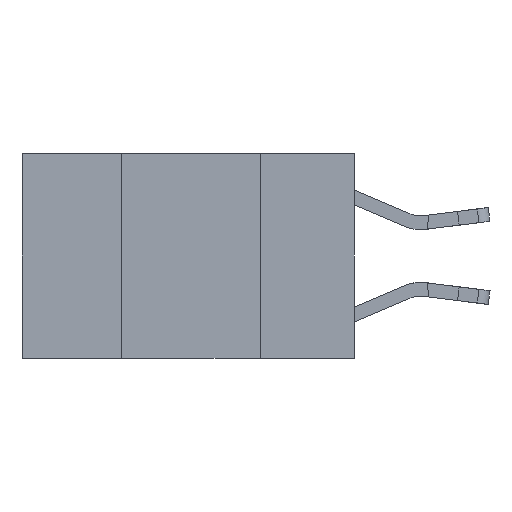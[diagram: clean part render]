
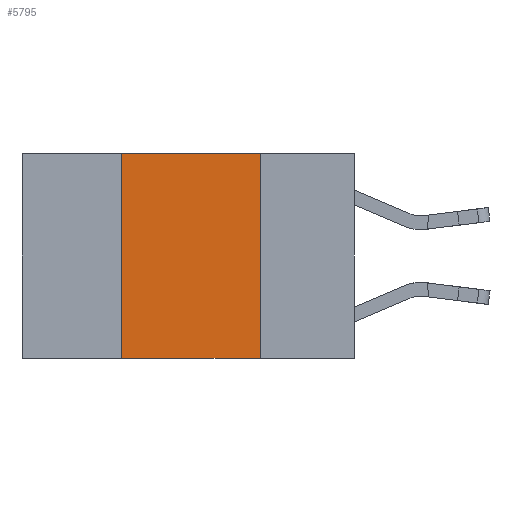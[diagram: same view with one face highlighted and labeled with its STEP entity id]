
A CAD part, left-side view. The second image highlights one B-rep face of the part: STEP entity #5795.
In plain terms, the highlighted planar face has unit normal (-1, 0, 0).
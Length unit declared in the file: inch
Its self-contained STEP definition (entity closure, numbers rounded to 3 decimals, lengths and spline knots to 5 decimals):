
#37 = CARTESIAN_POINT ( 'NONE',  ( 0., 0.42, 0. ) ) ;
#287 = PLANE ( 'NONE',  #8798 ) ;
#393 = DIRECTION ( 'NONE',  ( 0., -1., 0. ) ) ;
#747 = EDGE_CURVE ( 'NONE', #5703, #1092, #4711, .T. ) ;
#1092 = VERTEX_POINT ( 'NONE', #12671 ) ;
#2097 = VECTOR ( 'NONE', #13545, 39.37008 ) ;
#2302 = ORIENTED_EDGE ( 'NONE', *, *, #2569, .F. ) ;
#2569 = EDGE_CURVE ( 'NONE', #13637, #1092, #12019, .T. ) ;
#4104 = VECTOR ( 'NONE', #6028, 39.37008 ) ;
#4108 = DIRECTION ( 'NONE',  ( 1., 0., 0. ) ) ;
#4682 = CARTESIAN_POINT ( 'NONE',  ( 0., 0.42, 0. ) ) ;
#4711 = LINE ( 'NONE', #9185, #10938 ) ;
#4821 = FACE_OUTER_BOUND ( 'NONE', #12860, .T. ) ;
#4830 = CARTESIAN_POINT ( 'NONE',  ( 0., 0.17, 0. ) ) ;
#4950 = VECTOR ( 'NONE', #6341, 39.37008 ) ;
#4998 = ORIENTED_EDGE ( 'NONE', *, *, #747, .T. ) ;
#5330 = LINE ( 'NONE', #37, #4950 ) ;
#5703 = VERTEX_POINT ( 'NONE', #8920 ) ;
#5795 = ADVANCED_FACE ( 'NONE', ( #4821 ), #287, .F. ) ;
#6028 = DIRECTION ( 'NONE',  ( 0., -1., 0. ) ) ;
#6341 = DIRECTION ( 'NONE',  ( 0., 0., 1. ) ) ;
#7062 = CARTESIAN_POINT ( 'NONE',  ( 0., 0.17, 0. ) ) ;
#8798 = AXIS2_PLACEMENT_3D ( 'NONE', #9080, #4108, #12780 ) ;
#8920 = CARTESIAN_POINT ( 'NONE',  ( 0., 0.42, -0.37 ) ) ;
#9080 = CARTESIAN_POINT ( 'NONE',  ( 0., 0.6, 0. ) ) ;
#9185 = CARTESIAN_POINT ( 'NONE',  ( 0., 0.6, -0.37 ) ) ;
#10342 = LINE ( 'NONE', #12185, #4104 ) ;
#10938 = VECTOR ( 'NONE', #393, 39.37008 ) ;
#11125 = EDGE_CURVE ( 'NONE', #5703, #12873, #5330, .T. ) ;
#12019 = LINE ( 'NONE', #4830, #2097 ) ;
#12185 = CARTESIAN_POINT ( 'NONE',  ( 0., 0.6, 0. ) ) ;
#12671 = CARTESIAN_POINT ( 'NONE',  ( 0., 0.17, -0.37 ) ) ;
#12780 = DIRECTION ( 'NONE',  ( 0., 0., -1. ) ) ;
#12860 = EDGE_LOOP ( 'NONE', ( #2302, #13115, #14277, #4998 ) ) ;
#12873 = VERTEX_POINT ( 'NONE', #4682 ) ;
#13115 = ORIENTED_EDGE ( 'NONE', *, *, #13687, .F. ) ;
#13545 = DIRECTION ( 'NONE',  ( 0., 0., -1. ) ) ;
#13637 = VERTEX_POINT ( 'NONE', #7062 ) ;
#13687 = EDGE_CURVE ( 'NONE', #12873, #13637, #10342, .T. ) ;
#14277 = ORIENTED_EDGE ( 'NONE', *, *, #11125, .F. ) ;
